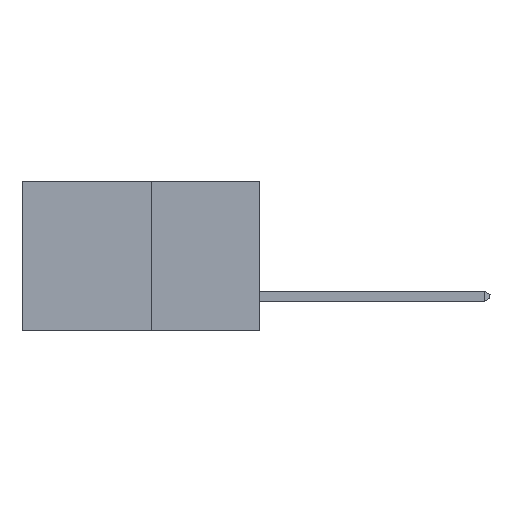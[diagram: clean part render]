
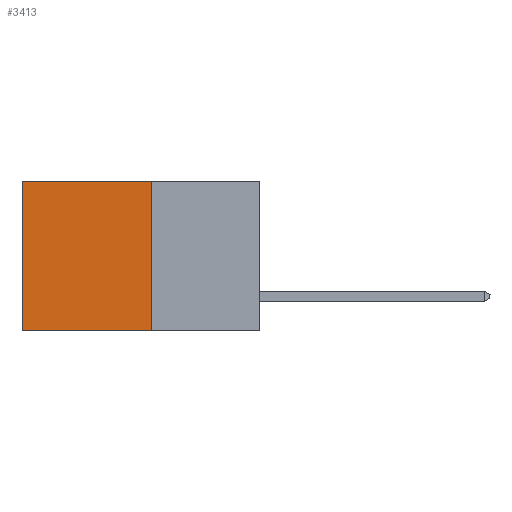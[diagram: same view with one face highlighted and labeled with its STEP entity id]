
A CAD part, left-side view. The second image highlights one B-rep face of the part: STEP entity #3413.
In plain terms, the highlighted planar face has unit normal (-1, 0, 0).
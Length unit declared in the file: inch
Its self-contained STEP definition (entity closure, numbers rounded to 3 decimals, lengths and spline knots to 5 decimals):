
#103 = VERTEX_POINT ( 'NONE', #4382 ) ;
#316 = CARTESIAN_POINT ( 'NONE',  ( 0.277, 0.27, 0. ) ) ;
#568 = ORIENTED_EDGE ( 'NONE', *, *, #2206, .F. ) ;
#883 = ORIENTED_EDGE ( 'NONE', *, *, #9548, .T. ) ;
#910 = DIRECTION ( 'NONE',  ( 1., 0., 0. ) ) ;
#956 = DIRECTION ( 'NONE',  ( 0., 1., 0. ) ) ;
#1345 = DIRECTION ( 'NONE',  ( 0., 0., -1. ) ) ;
#1695 = LINE ( 'NONE', #3958, #6032 ) ;
#2206 = EDGE_CURVE ( 'NONE', #103, #5313, #1695, .T. ) ;
#2848 = EDGE_CURVE ( 'NONE', #8997, #4684, #5804, .T. ) ;
#2970 = EDGE_CURVE ( 'NONE', #5313, #4684, #4571, .T. ) ;
#3413 = ADVANCED_FACE ( 'NONE', ( #5429 ), #7330, .F. ) ;
#3807 = DIRECTION ( 'NONE',  ( 0., 1., 0. ) ) ;
#3812 = AXIS2_PLACEMENT_3D ( 'NONE', #8212, #910, #1345 ) ;
#3958 = CARTESIAN_POINT ( 'NONE',  ( 0.277, 0.27, -0.37 ) ) ;
#4382 = CARTESIAN_POINT ( 'NONE',  ( 0.277, 0.27, 0. ) ) ;
#4571 = LINE ( 'NONE', #7991, #6596 ) ;
#4684 = VERTEX_POINT ( 'NONE', #9339 ) ;
#4818 = ORIENTED_EDGE ( 'NONE', *, *, #2970, .F. ) ;
#5313 = VERTEX_POINT ( 'NONE', #5384 ) ;
#5384 = CARTESIAN_POINT ( 'NONE',  ( 0.277, 0.27, -0.37 ) ) ;
#5429 = FACE_OUTER_BOUND ( 'NONE', #8530, .T. ) ;
#5544 = LINE ( 'NONE', #316, #7275 ) ;
#5804 = LINE ( 'NONE', #7005, #7514 ) ;
#6032 = VECTOR ( 'NONE', #9025, 39.37008 ) ;
#6479 = CARTESIAN_POINT ( 'NONE',  ( 0.277, 0.59, 0. ) ) ;
#6596 = VECTOR ( 'NONE', #956, 39.37008 ) ;
#7005 = CARTESIAN_POINT ( 'NONE',  ( 0.277, 0.59, -0.37 ) ) ;
#7049 = DIRECTION ( 'NONE',  ( 0., 0., -1. ) ) ;
#7275 = VECTOR ( 'NONE', #3807, 39.37008 ) ;
#7330 = PLANE ( 'NONE',  #3812 ) ;
#7514 = VECTOR ( 'NONE', #7049, 39.37008 ) ;
#7610 = ORIENTED_EDGE ( 'NONE', *, *, #2848, .T. ) ;
#7991 = CARTESIAN_POINT ( 'NONE',  ( 0.277, 0.27, -0.37 ) ) ;
#8212 = CARTESIAN_POINT ( 'NONE',  ( 0.277, 0.27, -0.37 ) ) ;
#8530 = EDGE_LOOP ( 'NONE', ( #7610, #4818, #568, #883 ) ) ;
#8997 = VERTEX_POINT ( 'NONE', #6479 ) ;
#9025 = DIRECTION ( 'NONE',  ( 0., 0., -1. ) ) ;
#9339 = CARTESIAN_POINT ( 'NONE',  ( 0.277, 0.59, -0.37 ) ) ;
#9548 = EDGE_CURVE ( 'NONE', #103, #8997, #5544, .T. ) ;
